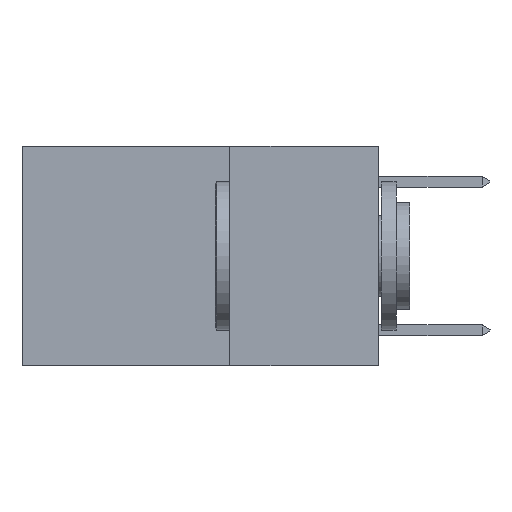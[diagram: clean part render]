
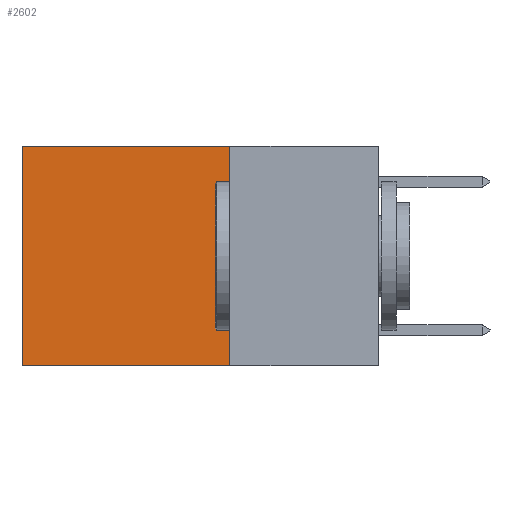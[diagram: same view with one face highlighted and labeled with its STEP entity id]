
A CAD part, left-side view. The second image highlights one B-rep face of the part: STEP entity #2602.
In plain terms, the highlighted planar face has unit normal (-1, 0, 0).
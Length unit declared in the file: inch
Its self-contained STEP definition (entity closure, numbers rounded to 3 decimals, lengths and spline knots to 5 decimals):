
#45 = VECTOR ( 'NONE', #8197, 39.37008 ) ;
#397 = CARTESIAN_POINT ( 'NONE',  ( 0.2625, 0.25, -0.37 ) ) ;
#986 = CARTESIAN_POINT ( 'NONE',  ( 0.2625, 0.25, 0. ) ) ;
#1063 = LINE ( 'NONE', #9319, #9441 ) ;
#1162 = VERTEX_POINT ( 'NONE', #7091 ) ;
#1380 = EDGE_CURVE ( 'NONE', #7503, #1162, #9736, .T. ) ;
#2325 = EDGE_CURVE ( 'NONE', #7503, #5223, #4737, .T. ) ;
#2391 = ORIENTED_EDGE ( 'NONE', *, *, #1380, .T. ) ;
#2602 = ADVANCED_FACE ( 'NONE', ( #10371 ), #5484, .F. ) ;
#2615 = ORIENTED_EDGE ( 'NONE', *, *, #3234, .T. ) ;
#2728 = VECTOR ( 'NONE', #8041, 39.37008 ) ;
#3234 = EDGE_CURVE ( 'NONE', #1162, #10357, #1063, .T. ) ;
#3282 = CARTESIAN_POINT ( 'NONE',  ( 0.2625, 0.25, 0. ) ) ;
#3705 = DIRECTION ( 'NONE',  ( 0., 1., 0. ) ) ;
#4313 = EDGE_CURVE ( 'NONE', #5223, #10357, #7427, .T. ) ;
#4715 = DIRECTION ( 'NONE',  ( 1., 0., 0. ) ) ;
#4737 = LINE ( 'NONE', #986, #2728 ) ;
#5160 = CARTESIAN_POINT ( 'NONE',  ( 0.2625, 0.25, 0. ) ) ;
#5223 = VERTEX_POINT ( 'NONE', #5785 ) ;
#5484 = PLANE ( 'NONE',  #8372 ) ;
#5785 = CARTESIAN_POINT ( 'NONE',  ( 0.2625, 0.25, -0.37 ) ) ;
#6300 = VECTOR ( 'NONE', #3705, 39.37008 ) ;
#6861 = ORIENTED_EDGE ( 'NONE', *, *, #4313, .F. ) ;
#7091 = CARTESIAN_POINT ( 'NONE',  ( 0.2625, 0.6, 0. ) ) ;
#7427 = LINE ( 'NONE', #397, #6300 ) ;
#7503 = VERTEX_POINT ( 'NONE', #5160 ) ;
#7953 = DIRECTION ( 'NONE',  ( 0., 0., -1. ) ) ;
#8041 = DIRECTION ( 'NONE',  ( 0., 0., -1. ) ) ;
#8197 = DIRECTION ( 'NONE',  ( 0., 1., 0. ) ) ;
#8372 = AXIS2_PLACEMENT_3D ( 'NONE', #8776, #4715, #9501 ) ;
#8622 = CARTESIAN_POINT ( 'NONE',  ( 0.2625, 0.6, -0.37 ) ) ;
#8776 = CARTESIAN_POINT ( 'NONE',  ( 0.2625, 0.25, 0. ) ) ;
#9152 = EDGE_LOOP ( 'NONE', ( #2615, #6861, #9489, #2391 ) ) ;
#9319 = CARTESIAN_POINT ( 'NONE',  ( 0.2625, 0.6, 0. ) ) ;
#9441 = VECTOR ( 'NONE', #7953, 39.37008 ) ;
#9489 = ORIENTED_EDGE ( 'NONE', *, *, #2325, .F. ) ;
#9501 = DIRECTION ( 'NONE',  ( 0., 0., -1. ) ) ;
#9736 = LINE ( 'NONE', #3282, #45 ) ;
#10357 = VERTEX_POINT ( 'NONE', #8622 ) ;
#10371 = FACE_OUTER_BOUND ( 'NONE', #9152, .T. ) ;
